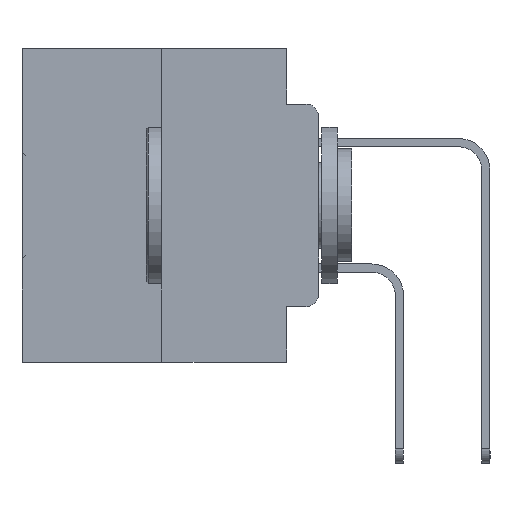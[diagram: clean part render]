
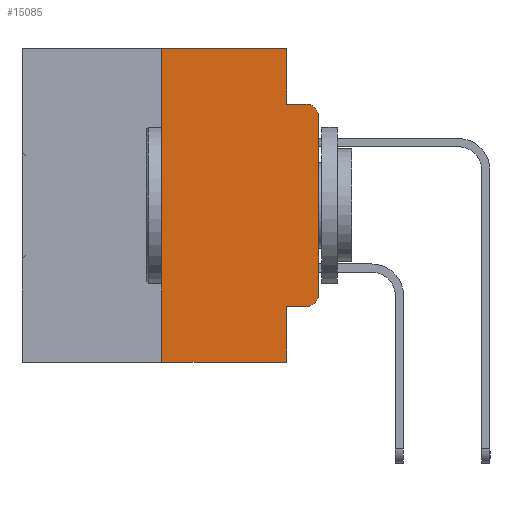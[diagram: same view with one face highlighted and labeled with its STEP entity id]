
A CAD part, left-side view. The second image highlights one B-rep face of the part: STEP entity #15085.
In plain terms, the highlighted planar face has unit normal (-1, 0, 0).
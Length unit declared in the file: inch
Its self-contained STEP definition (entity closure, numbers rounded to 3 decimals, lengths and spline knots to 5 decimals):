
#893 = ORIENTED_EDGE ( 'NONE', *, *, #19892, .F. ) ;
#1132 = ORIENTED_EDGE ( 'NONE', *, *, #33845, .T. ) ;
#1139 = ORIENTED_EDGE ( 'NONE', *, *, #32089, .T. ) ;
#1330 = CARTESIAN_POINT ( 'NONE',  ( 0., 0.473, -0.5 ) ) ;
#1430 = CARTESIAN_POINT ( 'NONE',  ( 0., 0.051, 0. ) ) ;
#1889 = CARTESIAN_POINT ( 'NONE',  ( 0., 0.02, -0.3915 ) ) ;
#2098 = LINE ( 'NONE', #4888, #20913 ) ;
#2226 = VECTOR ( 'NONE', #7877, 39.37008 ) ;
#2772 = CARTESIAN_POINT ( 'NONE',  ( 0., 0.25, 0. ) ) ;
#3311 = DIRECTION ( 'NONE',  ( 1., 0., 0. ) ) ;
#3344 = CARTESIAN_POINT ( 'NONE',  ( 0., 0.051, -0.4115 ) ) ;
#3397 = VERTEX_POINT ( 'NONE', #5887 ) ;
#4888 = CARTESIAN_POINT ( 'NONE',  ( 0., 0.051, -0.4115 ) ) ;
#5010 = CARTESIAN_POINT ( 'NONE',  ( 0., 0.051, -0.0885 ) ) ;
#5081 = CARTESIAN_POINT ( 'NONE',  ( 0., 0., 0. ) ) ;
#5187 = EDGE_CURVE ( 'NONE', #6277, #21134, #16386, .T. ) ;
#5393 = VECTOR ( 'NONE', #34281, 39.37008 ) ;
#5428 = CARTESIAN_POINT ( 'NONE',  ( 0., 0.473, 0. ) ) ;
#5736 = DIRECTION ( 'NONE',  ( 0., 0., 1. ) ) ;
#5852 = CARTESIAN_POINT ( 'NONE',  ( 0., 0., -0.1085 ) ) ;
#5876 = AXIS2_PLACEMENT_3D ( 'NONE', #5428, #3311, #27265 ) ;
#5887 = CARTESIAN_POINT ( 'NONE',  ( 0., 0.051, 0. ) ) ;
#5922 = ORIENTED_EDGE ( 'NONE', *, *, #26990, .T. ) ;
#5928 = VERTEX_POINT ( 'NONE', #6741 ) ;
#6277 = VERTEX_POINT ( 'NONE', #21910 ) ;
#6741 = CARTESIAN_POINT ( 'NONE',  ( 0., 0.02, -0.4115 ) ) ;
#7284 = LINE ( 'NONE', #23024, #19756 ) ;
#7710 = VERTEX_POINT ( 'NONE', #12133 ) ;
#7877 = DIRECTION ( 'NONE',  ( 0., 0., 1. ) ) ;
#8311 = CARTESIAN_POINT ( 'NONE',  ( 0., 0.02, -0.1085 ) ) ;
#9413 = CIRCLE ( 'NONE', #19412, 0.02 ) ;
#9484 = LINE ( 'NONE', #14538, #24149 ) ;
#9938 = VECTOR ( 'NONE', #25723, 39.37008 ) ;
#10372 = EDGE_CURVE ( 'NONE', #5928, #7710, #29061, .T. ) ;
#10383 = CARTESIAN_POINT ( 'NONE',  ( 0., 0.25, 0. ) ) ;
#10470 = DIRECTION ( 'NONE',  ( 0., 0., -1. ) ) ;
#10706 = EDGE_CURVE ( 'NONE', #6277, #12812, #25458, .T. ) ;
#11461 = CARTESIAN_POINT ( 'NONE',  ( 0., 0.051, -0.5 ) ) ;
#12133 = CARTESIAN_POINT ( 'NONE',  ( 0., 0., -0.3915 ) ) ;
#12812 = VERTEX_POINT ( 'NONE', #11461 ) ;
#14538 = CARTESIAN_POINT ( 'NONE',  ( 0., 0.051, 0. ) ) ;
#15085 = ADVANCED_FACE ( 'NONE', ( #32518 ), #29897, .F. ) ;
#15342 = DIRECTION ( 'NONE',  ( 0., 0., -1. ) ) ;
#15784 = VERTEX_POINT ( 'NONE', #5010 ) ;
#15904 = LINE ( 'NONE', #26578, #5393 ) ;
#16386 = LINE ( 'NONE', #2772, #26637 ) ;
#16732 = CARTESIAN_POINT ( 'NONE',  ( 0., 0.02, -0.0885 ) ) ;
#17215 = DIRECTION ( 'NONE',  ( 0., -1., 0. ) ) ;
#17938 = ORIENTED_EDGE ( 'NONE', *, *, #18763, .F. ) ;
#18763 = EDGE_CURVE ( 'NONE', #21134, #3397, #15904, .T. ) ;
#19412 = AXIS2_PLACEMENT_3D ( 'NONE', #8311, #30152, #10470 ) ;
#19756 = VECTOR ( 'NONE', #33686, 39.37008 ) ;
#19892 = EDGE_CURVE ( 'NONE', #3397, #15784, #22746, .T. ) ;
#20387 = ORIENTED_EDGE ( 'NONE', *, *, #10706, .T. ) ;
#20913 = VECTOR ( 'NONE', #26226, 39.37008 ) ;
#21134 = VERTEX_POINT ( 'NONE', #10383 ) ;
#21910 = CARTESIAN_POINT ( 'NONE',  ( 0., 0.25, -0.5 ) ) ;
#22341 = ORIENTED_EDGE ( 'NONE', *, *, #10372, .T. ) ;
#22746 = LINE ( 'NONE', #1430, #9938 ) ;
#22790 = EDGE_CURVE ( 'NONE', #33457, #12812, #9484, .T. ) ;
#22921 = VECTOR ( 'NONE', #17215, 39.37008 ) ;
#22976 = EDGE_LOOP ( 'NONE', ( #1132, #1139, #30637, #893, #17938, #25359, #20387, #32824, #5922, #22341 ) ) ;
#23024 = CARTESIAN_POINT ( 'NONE',  ( 0., 0.051, -0.0885 ) ) ;
#23223 = DIRECTION ( 'NONE',  ( -1., 0., 0. ) ) ;
#24149 = VECTOR ( 'NONE', #33942, 39.37008 ) ;
#24846 = EDGE_CURVE ( 'NONE', #15784, #27205, #7284, .T. ) ;
#25359 = ORIENTED_EDGE ( 'NONE', *, *, #5187, .F. ) ;
#25458 = LINE ( 'NONE', #1330, #22921 ) ;
#25723 = DIRECTION ( 'NONE',  ( 0., 0., -1. ) ) ;
#26226 = DIRECTION ( 'NONE',  ( 0., -1., 0. ) ) ;
#26578 = CARTESIAN_POINT ( 'NONE',  ( 0., 0.473, 0. ) ) ;
#26637 = VECTOR ( 'NONE', #5736, 39.37008 ) ;
#26990 = EDGE_CURVE ( 'NONE', #33457, #5928, #2098, .T. ) ;
#27205 = VERTEX_POINT ( 'NONE', #16732 ) ;
#27265 = DIRECTION ( 'NONE',  ( 0., 0., -1. ) ) ;
#27930 = AXIS2_PLACEMENT_3D ( 'NONE', #1889, #23223, #15342 ) ;
#29061 = CIRCLE ( 'NONE', #27930, 0.02 ) ;
#29416 = VERTEX_POINT ( 'NONE', #5852 ) ;
#29897 = PLANE ( 'NONE',  #5876 ) ;
#30152 = DIRECTION ( 'NONE',  ( -1., 0., 0. ) ) ;
#30637 = ORIENTED_EDGE ( 'NONE', *, *, #24846, .F. ) ;
#31496 = LINE ( 'NONE', #5081, #2226 ) ;
#32089 = EDGE_CURVE ( 'NONE', #29416, #27205, #9413, .T. ) ;
#32518 = FACE_OUTER_BOUND ( 'NONE', #22976, .T. ) ;
#32824 = ORIENTED_EDGE ( 'NONE', *, *, #22790, .F. ) ;
#33457 = VERTEX_POINT ( 'NONE', #3344 ) ;
#33686 = DIRECTION ( 'NONE',  ( 0., -1., 0. ) ) ;
#33845 = EDGE_CURVE ( 'NONE', #7710, #29416, #31496, .T. ) ;
#33942 = DIRECTION ( 'NONE',  ( 0., 0., -1. ) ) ;
#34281 = DIRECTION ( 'NONE',  ( 0., -1., 0. ) ) ;
